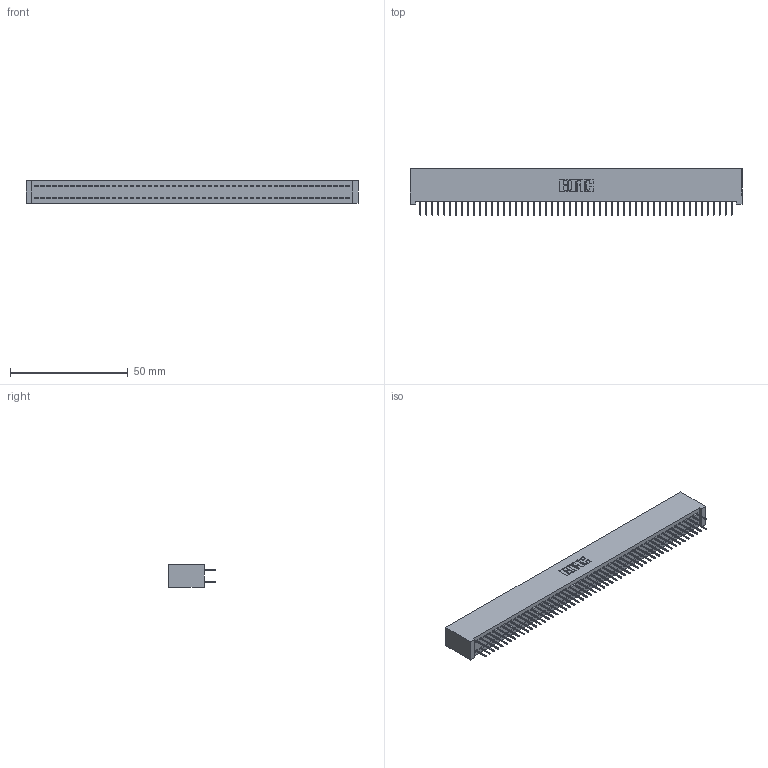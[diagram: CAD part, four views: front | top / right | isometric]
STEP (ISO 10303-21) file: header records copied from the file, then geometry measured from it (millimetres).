
FILE_DESCRIPTION (( 'STEP AP203' ), '1' );
FILE_NAME ('342-106-524-201.STEP', '2019-10-04T19:09:04', ( '' ), ( '' ), 'SwSTEP 2.0', 'SolidWorks 2016', '' );
FILE_SCHEMA (( 'CONFIG_CONTROL_DESIGN' ));
Length unit declared in the file: inch
Products named in the file (3): 342 Part_Lugless; 345-292-001_345-293-124; 342-106-524-201
Assembly tree (107 placements, depth 2):
  342-106-524-201
    342 Part_Lugless
    345-292-001_345-293-124  x106
Bounding box: 140.87 x 19.69 x 9.4 mm (x, y, z)
Volume: 12988.2 mm3; surface area: 21441.5 mm2
Topology: 107 solids, 107 shells, 6038 faces, 17129 edges, 10994 vertices
Faces by surface type: plane 4514, cylinder 1524
Entity records: 32339 total; most frequent: CARTESIAN_POINT 5342, ORIENTED_EDGE 5278, DIRECTION 4539, EDGE_CURVE 2639, VECTOR 2523, LINE 2523, VERTEX_POINT 1754, AXIS2_PLACEMENT_3D 1008
